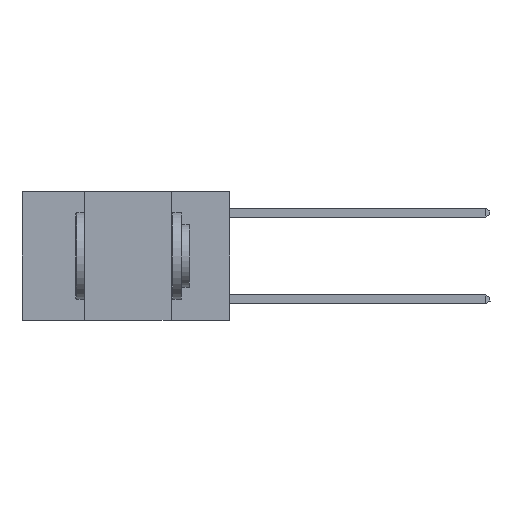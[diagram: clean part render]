
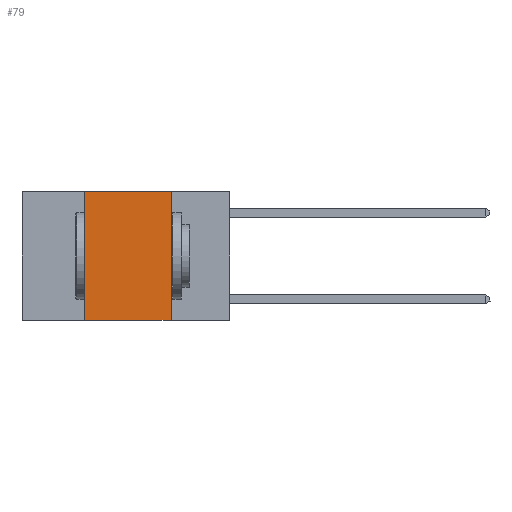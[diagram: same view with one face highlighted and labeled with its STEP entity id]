
A CAD part, left-side view. The second image highlights one B-rep face of the part: STEP entity #79.
In plain terms, the highlighted planar face has unit normal (-1, 0, 0).
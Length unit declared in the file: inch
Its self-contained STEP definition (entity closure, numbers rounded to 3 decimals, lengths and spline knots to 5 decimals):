
#79 = ADVANCED_FACE ( 'NONE', ( #21996 ), #32096, .F. ) ;
#160 = VECTOR ( 'NONE', #10538, 39.37008 ) ;
#1904 = CARTESIAN_POINT ( 'NONE',  ( 0., 0.17, 0. ) ) ;
#2192 = VERTEX_POINT ( 'NONE', #18884 ) ;
#3032 = VECTOR ( 'NONE', #10095, 39.37008 ) ;
#4322 = CARTESIAN_POINT ( 'NONE',  ( 0., 0.42, -0.37 ) ) ;
#4620 = VERTEX_POINT ( 'NONE', #11874 ) ;
#6883 = DIRECTION ( 'NONE',  ( 1., 0., 0. ) ) ;
#7033 = EDGE_CURVE ( 'NONE', #18694, #4620, #22887, .T. ) ;
#7096 = EDGE_CURVE ( 'NONE', #4620, #18347, #28049, .T. ) ;
#9575 = LINE ( 'NONE', #1904, #23473 ) ;
#9857 = EDGE_CURVE ( 'NONE', #18694, #2192, #23836, .T. ) ;
#10095 = DIRECTION ( 'NONE',  ( 0., -1., 0. ) ) ;
#10538 = DIRECTION ( 'NONE',  ( 0., -1., 0. ) ) ;
#11874 = CARTESIAN_POINT ( 'NONE',  ( 0., 0.42, 0. ) ) ;
#15498 = CARTESIAN_POINT ( 'NONE',  ( 0., 0.6, -0.37 ) ) ;
#17029 = DIRECTION ( 'NONE',  ( 0., 0., -1. ) ) ;
#17281 = AXIS2_PLACEMENT_3D ( 'NONE', #29645, #6883, #17029 ) ;
#17577 = CARTESIAN_POINT ( 'NONE',  ( 0., 0.6, 0. ) ) ;
#18252 = EDGE_CURVE ( 'NONE', #18347, #2192, #9575, .T. ) ;
#18347 = VERTEX_POINT ( 'NONE', #25170 ) ;
#18694 = VERTEX_POINT ( 'NONE', #4322 ) ;
#18884 = CARTESIAN_POINT ( 'NONE',  ( 0., 0.17, -0.37 ) ) ;
#19333 = ORIENTED_EDGE ( 'NONE', *, *, #18252, .F. ) ;
#21996 = FACE_OUTER_BOUND ( 'NONE', #29895, .T. ) ;
#22887 = LINE ( 'NONE', #25206, #23782 ) ;
#23473 = VECTOR ( 'NONE', #24544, 39.37008 ) ;
#23782 = VECTOR ( 'NONE', #30334, 39.37008 ) ;
#23836 = LINE ( 'NONE', #15498, #160 ) ;
#24544 = DIRECTION ( 'NONE',  ( 0., 0., -1. ) ) ;
#25119 = ORIENTED_EDGE ( 'NONE', *, *, #9857, .T. ) ;
#25170 = CARTESIAN_POINT ( 'NONE',  ( 0., 0.17, 0. ) ) ;
#25187 = ORIENTED_EDGE ( 'NONE', *, *, #7033, .F. ) ;
#25206 = CARTESIAN_POINT ( 'NONE',  ( 0., 0.42, 0. ) ) ;
#28049 = LINE ( 'NONE', #17577, #3032 ) ;
#28997 = ORIENTED_EDGE ( 'NONE', *, *, #7096, .F. ) ;
#29645 = CARTESIAN_POINT ( 'NONE',  ( 0., 0.6, 0. ) ) ;
#29895 = EDGE_LOOP ( 'NONE', ( #19333, #28997, #25187, #25119 ) ) ;
#30334 = DIRECTION ( 'NONE',  ( 0., 0., 1. ) ) ;
#32096 = PLANE ( 'NONE',  #17281 ) ;
